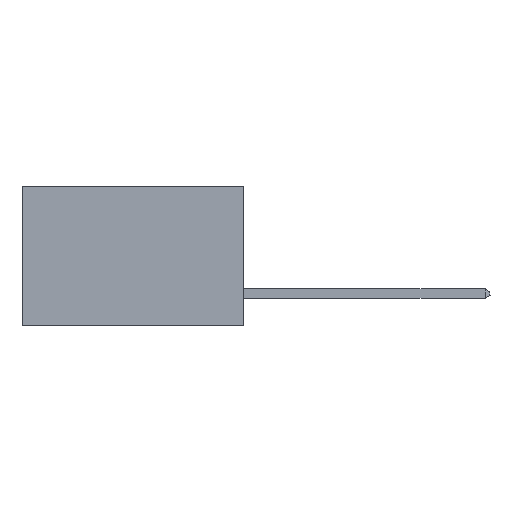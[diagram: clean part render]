
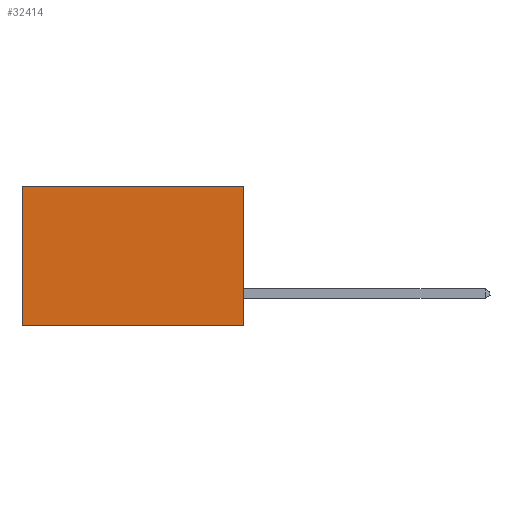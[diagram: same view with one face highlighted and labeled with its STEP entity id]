
A CAD part, left-side view. The second image highlights one B-rep face of the part: STEP entity #32414.
In plain terms, the highlighted planar face has unit normal (-1, 0, 0).
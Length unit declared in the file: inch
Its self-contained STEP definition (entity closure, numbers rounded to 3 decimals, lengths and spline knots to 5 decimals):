
#1033 = CARTESIAN_POINT ( 'NONE',  ( 0.277, 0., -0.37 ) ) ;
#1640 = ORIENTED_EDGE ( 'NONE', *, *, #20640, .T. ) ;
#1766 = ORIENTED_EDGE ( 'NONE', *, *, #2523, .F. ) ;
#2523 = EDGE_CURVE ( 'NONE', #24559, #24730, #20984, .T. ) ;
#2905 = LINE ( 'NONE', #32372, #8857 ) ;
#3597 = DIRECTION ( 'NONE',  ( 0., 0., -1. ) ) ;
#4280 = CARTESIAN_POINT ( 'NONE',  ( 0.277, 0.59, 0. ) ) ;
#7748 = ORIENTED_EDGE ( 'NONE', *, *, #28932, .F. ) ;
#7837 = EDGE_LOOP ( 'NONE', ( #1640, #1766, #7748, #14387 ) ) ;
#8857 = VECTOR ( 'NONE', #14616, 39.37008 ) ;
#8932 = VECTOR ( 'NONE', #11051, 39.37008 ) ;
#9478 = CARTESIAN_POINT ( 'NONE',  ( 0.277, 0.59, -0.37 ) ) ;
#11051 = DIRECTION ( 'NONE',  ( 0., 1., 0. ) ) ;
#13131 = VECTOR ( 'NONE', #30390, 39.37008 ) ;
#13231 = LINE ( 'NONE', #27125, #27617 ) ;
#14387 = ORIENTED_EDGE ( 'NONE', *, *, #16534, .T. ) ;
#14616 = DIRECTION ( 'NONE',  ( 0., 0., -1. ) ) ;
#16345 = PLANE ( 'NONE',  #16658 ) ;
#16534 = EDGE_CURVE ( 'NONE', #28678, #18991, #19941, .T. ) ;
#16658 = AXIS2_PLACEMENT_3D ( 'NONE', #1033, #18907, #3597 ) ;
#18907 = DIRECTION ( 'NONE',  ( 1., 0., 0. ) ) ;
#18991 = VERTEX_POINT ( 'NONE', #4280 ) ;
#19941 = LINE ( 'NONE', #32890, #13131 ) ;
#20640 = EDGE_CURVE ( 'NONE', #18991, #24730, #13231, .T. ) ;
#20984 = LINE ( 'NONE', #26972, #8932 ) ;
#24559 = VERTEX_POINT ( 'NONE', #29240 ) ;
#24730 = VERTEX_POINT ( 'NONE', #9478 ) ;
#26972 = CARTESIAN_POINT ( 'NONE',  ( 0.277, 0., -0.37 ) ) ;
#27125 = CARTESIAN_POINT ( 'NONE',  ( 0.277, 0.59, -0.37 ) ) ;
#27617 = VECTOR ( 'NONE', #29623, 39.37008 ) ;
#28678 = VERTEX_POINT ( 'NONE', #31377 ) ;
#28932 = EDGE_CURVE ( 'NONE', #28678, #24559, #2905, .T. ) ;
#29240 = CARTESIAN_POINT ( 'NONE',  ( 0.277, 0., -0.37 ) ) ;
#29623 = DIRECTION ( 'NONE',  ( 0., 0., -1. ) ) ;
#30390 = DIRECTION ( 'NONE',  ( 0., 1., 0. ) ) ;
#30910 = FACE_OUTER_BOUND ( 'NONE', #7837, .T. ) ;
#31377 = CARTESIAN_POINT ( 'NONE',  ( 0.277, 0., 0. ) ) ;
#32372 = CARTESIAN_POINT ( 'NONE',  ( 0.277, 0., -0.37 ) ) ;
#32414 = ADVANCED_FACE ( 'NONE', ( #30910 ), #16345, .F. ) ;
#32890 = CARTESIAN_POINT ( 'NONE',  ( 0.277, 0., 0. ) ) ;
